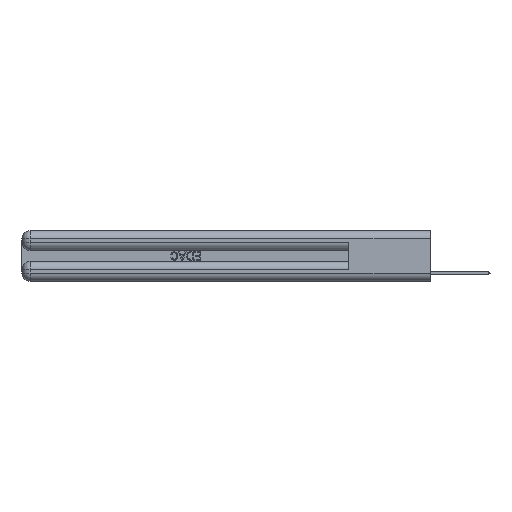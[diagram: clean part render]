
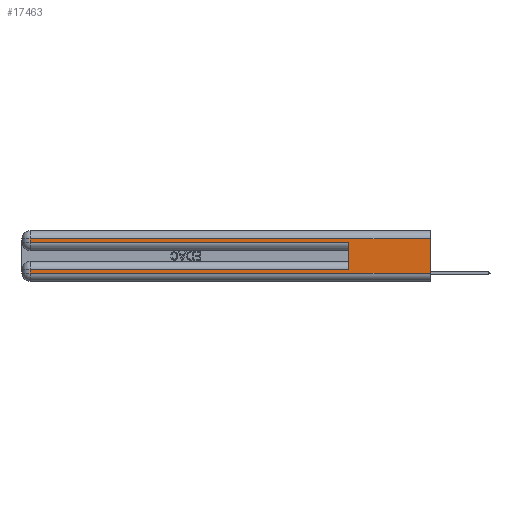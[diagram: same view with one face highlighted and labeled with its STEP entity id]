
A CAD part, left-side view. The second image highlights one B-rep face of the part: STEP entity #17463.
In plain terms, the highlighted planar face has unit normal (-1, 0, 0).
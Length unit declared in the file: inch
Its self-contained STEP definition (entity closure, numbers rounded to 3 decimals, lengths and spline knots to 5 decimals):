
#347 = VERTEX_POINT ( 'NONE', #24932 ) ;
#400 = LINE ( 'NONE', #6647, #25202 ) ;
#1246 = DIRECTION ( 'NONE',  ( 0., 0., 1. ) ) ;
#1349 = DIRECTION ( 'NONE',  ( 0., 1., 0. ) ) ;
#1603 = ORIENTED_EDGE ( 'NONE', *, *, #14759, .T. ) ;
#1918 = DIRECTION ( 'NONE',  ( 0., -1., 0. ) ) ;
#2071 = CARTESIAN_POINT ( 'NONE',  ( 0., 2.94, 0.085 ) ) ;
#2903 = CARTESIAN_POINT ( 'NONE',  ( 0., 0., 0.37 ) ) ;
#3682 = VECTOR ( 'NONE', #12077, 39.37008 ) ;
#3903 = DIRECTION ( 'NONE',  ( 1., 0., 0. ) ) ;
#4299 = LINE ( 'NONE', #12571, #12159 ) ;
#5418 = CARTESIAN_POINT ( 'NONE',  ( 0., 0., 0.31 ) ) ;
#5850 = CARTESIAN_POINT ( 'NONE',  ( 0., 2.94, 0.37 ) ) ;
#6647 = CARTESIAN_POINT ( 'NONE',  ( 0., 0., 0.285 ) ) ;
#7409 = VERTEX_POINT ( 'NONE', #16731 ) ;
#8933 = CARTESIAN_POINT ( 'NONE',  ( 0., 0., 0.37 ) ) ;
#9084 = LINE ( 'NONE', #23489, #23313 ) ;
#9711 = EDGE_CURVE ( 'NONE', #17125, #13089, #25430, .T. ) ;
#9994 = VERTEX_POINT ( 'NONE', #2071 ) ;
#10219 = EDGE_LOOP ( 'NONE', ( #13479, #25253, #12521, #1603, #24898, #23315, #10378, #16618 ) ) ;
#10378 = ORIENTED_EDGE ( 'NONE', *, *, #11545, .T. ) ;
#10572 = CARTESIAN_POINT ( 'NONE',  ( 0., 0.6, 0.285 ) ) ;
#11415 = AXIS2_PLACEMENT_3D ( 'NONE', #8933, #3903, #24540 ) ;
#11494 = FACE_OUTER_BOUND ( 'NONE', #10219, .T. ) ;
#11545 = EDGE_CURVE ( 'NONE', #9994, #12980, #22664, .T. ) ;
#12071 = EDGE_CURVE ( 'NONE', #7409, #9994, #4299, .T. ) ;
#12077 = DIRECTION ( 'NONE',  ( 0., 0., -1. ) ) ;
#12141 = VECTOR ( 'NONE', #12468, 39.37008 ) ;
#12159 = VECTOR ( 'NONE', #20595, 39.37008 ) ;
#12460 = VERTEX_POINT ( 'NONE', #12699 ) ;
#12468 = DIRECTION ( 'NONE',  ( 0., 0., -1. ) ) ;
#12521 = ORIENTED_EDGE ( 'NONE', *, *, #18399, .T. ) ;
#12571 = CARTESIAN_POINT ( 'NONE',  ( 0., 0., 0.085 ) ) ;
#12699 = CARTESIAN_POINT ( 'NONE',  ( 0., 2.94, 0.31 ) ) ;
#12949 = VECTOR ( 'NONE', #1349, 39.37008 ) ;
#12980 = VERTEX_POINT ( 'NONE', #20827 ) ;
#13089 = VERTEX_POINT ( 'NONE', #13603 ) ;
#13479 = ORIENTED_EDGE ( 'NONE', *, *, #9711, .F. ) ;
#13596 = DIRECTION ( 'NONE',  ( 0., 0., -1. ) ) ;
#13603 = CARTESIAN_POINT ( 'NONE',  ( 0., 0., 0.06 ) ) ;
#14083 = LINE ( 'NONE', #5418, #12949 ) ;
#14759 = EDGE_CURVE ( 'NONE', #347, #14880, #400, .T. ) ;
#14880 = VERTEX_POINT ( 'NONE', #10572 ) ;
#15480 = LINE ( 'NONE', #23767, #16131 ) ;
#15852 = EDGE_CURVE ( 'NONE', #7409, #14880, #15480, .T. ) ;
#16131 = VECTOR ( 'NONE', #1246, 39.37008 ) ;
#16618 = ORIENTED_EDGE ( 'NONE', *, *, #23523, .T. ) ;
#16731 = CARTESIAN_POINT ( 'NONE',  ( 0., 0.6, 0.085 ) ) ;
#17125 = VERTEX_POINT ( 'NONE', #20090 ) ;
#17229 = DIRECTION ( 'NONE',  ( 0., -1., 0. ) ) ;
#17463 = ADVANCED_FACE ( 'NONE', ( #11494 ), #19783, .F. ) ;
#18330 = LINE ( 'NONE', #5850, #3682 ) ;
#18399 = EDGE_CURVE ( 'NONE', #12460, #347, #18330, .T. ) ;
#18590 = CARTESIAN_POINT ( 'NONE',  ( 0., 2.94, 0.37 ) ) ;
#19445 = VECTOR ( 'NONE', #13596, 39.37008 ) ;
#19783 = PLANE ( 'NONE',  #11415 ) ;
#20090 = CARTESIAN_POINT ( 'NONE',  ( 0., 0., 0.31 ) ) ;
#20595 = DIRECTION ( 'NONE',  ( 0., 1., 0. ) ) ;
#20827 = CARTESIAN_POINT ( 'NONE',  ( 0., 2.94, 0.06 ) ) ;
#22664 = LINE ( 'NONE', #18590, #12141 ) ;
#23313 = VECTOR ( 'NONE', #17229, 39.37008 ) ;
#23315 = ORIENTED_EDGE ( 'NONE', *, *, #12071, .T. ) ;
#23489 = CARTESIAN_POINT ( 'NONE',  ( 0., 0., 0.06 ) ) ;
#23523 = EDGE_CURVE ( 'NONE', #12980, #13089, #9084, .T. ) ;
#23767 = CARTESIAN_POINT ( 'NONE',  ( 0., 0.6, 0.145 ) ) ;
#24540 = DIRECTION ( 'NONE',  ( 0., 0., -1. ) ) ;
#24898 = ORIENTED_EDGE ( 'NONE', *, *, #15852, .F. ) ;
#24932 = CARTESIAN_POINT ( 'NONE',  ( 0., 2.94, 0.285 ) ) ;
#25202 = VECTOR ( 'NONE', #1918, 39.37008 ) ;
#25253 = ORIENTED_EDGE ( 'NONE', *, *, #26687, .T. ) ;
#25430 = LINE ( 'NONE', #2903, #19445 ) ;
#26687 = EDGE_CURVE ( 'NONE', #17125, #12460, #14083, .T. ) ;
